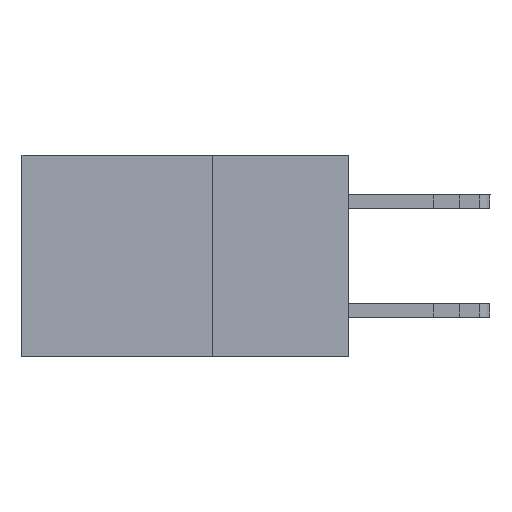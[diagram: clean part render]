
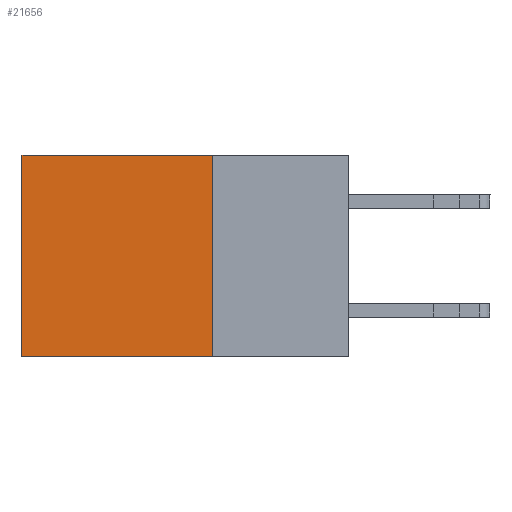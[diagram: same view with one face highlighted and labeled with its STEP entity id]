
A CAD part, left-side view. The second image highlights one B-rep face of the part: STEP entity #21656.
In plain terms, the highlighted planar face has unit normal (-1, 0, 0).
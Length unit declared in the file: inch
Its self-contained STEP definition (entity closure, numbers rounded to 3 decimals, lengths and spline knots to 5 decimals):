
#84 = VERTEX_POINT ( 'NONE', #6414 ) ;
#386 = VECTOR ( 'NONE', #7798, 39.37008 ) ;
#592 = VECTOR ( 'NONE', #18887, 39.37008 ) ;
#1365 = CARTESIAN_POINT ( 'NONE',  ( 0.298, 0.25, 0. ) ) ;
#1436 = CARTESIAN_POINT ( 'NONE',  ( 0.298, 0.6, 0. ) ) ;
#1502 = EDGE_CURVE ( 'NONE', #22637, #7282, #6048, .T. ) ;
#1756 = VERTEX_POINT ( 'NONE', #10883 ) ;
#1892 = ORIENTED_EDGE ( 'NONE', *, *, #21835, .T. ) ;
#1930 = EDGE_CURVE ( 'NONE', #22637, #84, #9808, .T. ) ;
#3661 = EDGE_CURVE ( 'NONE', #7282, #1756, #7893, .T. ) ;
#6048 = LINE ( 'NONE', #13035, #8260 ) ;
#6114 = CARTESIAN_POINT ( 'NONE',  ( 0.298, 0.25, -0.37 ) ) ;
#6414 = CARTESIAN_POINT ( 'NONE',  ( 0.298, 0.6, 0. ) ) ;
#6711 = VECTOR ( 'NONE', #7237, 39.37008 ) ;
#7237 = DIRECTION ( 'NONE',  ( 0., 0., -1. ) ) ;
#7282 = VERTEX_POINT ( 'NONE', #18368 ) ;
#7798 = DIRECTION ( 'NONE',  ( 0., 1., 0. ) ) ;
#7893 = LINE ( 'NONE', #6114, #592 ) ;
#8260 = VECTOR ( 'NONE', #20235, 39.37008 ) ;
#8585 = DIRECTION ( 'NONE',  ( 1., 0., 0. ) ) ;
#9808 = LINE ( 'NONE', #13241, #386 ) ;
#10127 = AXIS2_PLACEMENT_3D ( 'NONE', #1365, #8585, #10493 ) ;
#10493 = DIRECTION ( 'NONE',  ( 0., 0., -1. ) ) ;
#10611 = PLANE ( 'NONE',  #10127 ) ;
#10883 = CARTESIAN_POINT ( 'NONE',  ( 0.298, 0.6, -0.37 ) ) ;
#13035 = CARTESIAN_POINT ( 'NONE',  ( 0.298, 0.25, 0. ) ) ;
#13241 = CARTESIAN_POINT ( 'NONE',  ( 0.298, 0.25, 0. ) ) ;
#14108 = ORIENTED_EDGE ( 'NONE', *, *, #1930, .T. ) ;
#14206 = ORIENTED_EDGE ( 'NONE', *, *, #1502, .F. ) ;
#14516 = ORIENTED_EDGE ( 'NONE', *, *, #3661, .F. ) ;
#15853 = EDGE_LOOP ( 'NONE', ( #1892, #14516, #14206, #14108 ) ) ;
#16180 = FACE_OUTER_BOUND ( 'NONE', #15853, .T. ) ;
#17409 = CARTESIAN_POINT ( 'NONE',  ( 0.298, 0.25, 0. ) ) ;
#17661 = LINE ( 'NONE', #1436, #6711 ) ;
#18368 = CARTESIAN_POINT ( 'NONE',  ( 0.298, 0.25, -0.37 ) ) ;
#18887 = DIRECTION ( 'NONE',  ( 0., 1., 0. ) ) ;
#20235 = DIRECTION ( 'NONE',  ( 0., 0., -1. ) ) ;
#21656 = ADVANCED_FACE ( 'NONE', ( #16180 ), #10611, .F. ) ;
#21835 = EDGE_CURVE ( 'NONE', #84, #1756, #17661, .T. ) ;
#22637 = VERTEX_POINT ( 'NONE', #17409 ) ;
